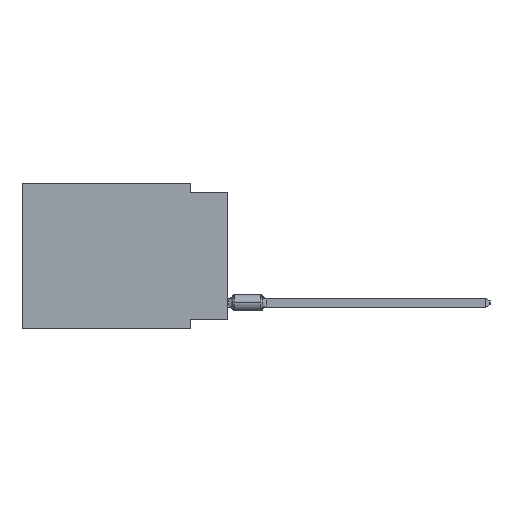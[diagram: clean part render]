
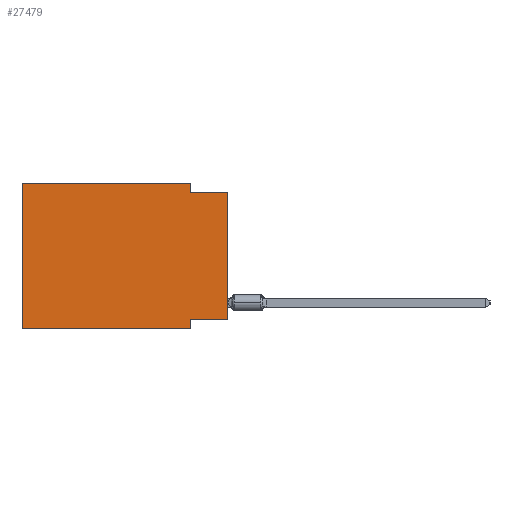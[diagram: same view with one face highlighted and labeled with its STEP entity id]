
A CAD part, left-side view. The second image highlights one B-rep face of the part: STEP entity #27479.
In plain terms, the highlighted planar face has unit normal (-1, 0, 0).
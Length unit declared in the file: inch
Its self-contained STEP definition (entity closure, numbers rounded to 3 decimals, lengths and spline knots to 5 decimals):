
#894 = VERTEX_POINT ( 'NONE', #2018 ) ;
#1038 = ORIENTED_EDGE ( 'NONE', *, *, #21300, .F. ) ;
#1044 = EDGE_CURVE ( 'NONE', #894, #15032, #33565, .T. ) ;
#1899 = DIRECTION ( 'NONE',  ( 0., -1., 0. ) ) ;
#1952 = LINE ( 'NONE', #21117, #22006 ) ;
#2018 = CARTESIAN_POINT ( 'NONE',  ( 0., 0.1, 0. ) ) ;
#2833 = EDGE_CURVE ( 'NONE', #34640, #15910, #15839, .T. ) ;
#4750 = VERTEX_POINT ( 'NONE', #22282 ) ;
#5182 = CARTESIAN_POINT ( 'NONE',  ( 0., 0.55, -0.39 ) ) ;
#5413 = DIRECTION ( 'NONE',  ( 0., 1., 0. ) ) ;
#6310 = VECTOR ( 'NONE', #17006, 39.37008 ) ;
#6360 = VECTOR ( 'NONE', #30102, 39.37008 ) ;
#6631 = CARTESIAN_POINT ( 'NONE',  ( 0., 0.55, 0. ) ) ;
#6799 = EDGE_CURVE ( 'NONE', #15032, #14918, #14564, .T. ) ;
#6900 = CARTESIAN_POINT ( 'NONE',  ( 0., 0.1, -0.39 ) ) ;
#7447 = VERTEX_POINT ( 'NONE', #28663 ) ;
#7668 = CARTESIAN_POINT ( 'NONE',  ( 0., 0.1, -0.365 ) ) ;
#8268 = ORIENTED_EDGE ( 'NONE', *, *, #36046, .F. ) ;
#8317 = LINE ( 'NONE', #19436, #23651 ) ;
#8436 = ORIENTED_EDGE ( 'NONE', *, *, #2833, .F. ) ;
#9381 = FACE_OUTER_BOUND ( 'NONE', #31543, .T. ) ;
#11258 = EDGE_CURVE ( 'NONE', #7447, #15910, #35103, .T. ) ;
#12214 = ORIENTED_EDGE ( 'NONE', *, *, #6799, .F. ) ;
#12831 = DIRECTION ( 'NONE',  ( 1., 0., 0. ) ) ;
#13081 = DIRECTION ( 'NONE',  ( 0., 0., 1. ) ) ;
#14133 = ORIENTED_EDGE ( 'NONE', *, *, #23412, .T. ) ;
#14235 = CARTESIAN_POINT ( 'NONE',  ( 0., 0.1, 0. ) ) ;
#14552 = VECTOR ( 'NONE', #5413, 39.37008 ) ;
#14564 = LINE ( 'NONE', #22567, #31024 ) ;
#14719 = CARTESIAN_POINT ( 'NONE',  ( 0., 0.55, 0. ) ) ;
#14918 = VERTEX_POINT ( 'NONE', #34698 ) ;
#15032 = VERTEX_POINT ( 'NONE', #18269 ) ;
#15839 = LINE ( 'NONE', #21483, #21558 ) ;
#15910 = VERTEX_POINT ( 'NONE', #6900 ) ;
#16382 = LINE ( 'NONE', #30757, #14552 ) ;
#17006 = DIRECTION ( 'NONE',  ( 0., -1., 0. ) ) ;
#18269 = CARTESIAN_POINT ( 'NONE',  ( 0., 0.1, -0.025 ) ) ;
#18277 = ORIENTED_EDGE ( 'NONE', *, *, #29697, .F. ) ;
#18295 = ORIENTED_EDGE ( 'NONE', *, *, #1044, .F. ) ;
#18969 = VECTOR ( 'NONE', #1899, 39.37008 ) ;
#19436 = CARTESIAN_POINT ( 'NONE',  ( 0., 0.55, 0. ) ) ;
#21117 = CARTESIAN_POINT ( 'NONE',  ( 0., 0., 0. ) ) ;
#21300 = EDGE_CURVE ( 'NONE', #7447, #21398, #8317, .T. ) ;
#21398 = VERTEX_POINT ( 'NONE', #14719 ) ;
#21483 = CARTESIAN_POINT ( 'NONE',  ( 0., 0.1, -0.39 ) ) ;
#21558 = VECTOR ( 'NONE', #23678, 39.37008 ) ;
#22006 = VECTOR ( 'NONE', #13081, 39.37008 ) ;
#22282 = CARTESIAN_POINT ( 'NONE',  ( 0., 0., -0.365 ) ) ;
#22567 = CARTESIAN_POINT ( 'NONE',  ( 0., 0., -0.025 ) ) ;
#23412 = EDGE_CURVE ( 'NONE', #4750, #14918, #1952, .T. ) ;
#23651 = VECTOR ( 'NONE', #30550, 39.37008 ) ;
#23678 = DIRECTION ( 'NONE',  ( 0., 0., -1. ) ) ;
#23954 = DIRECTION ( 'NONE',  ( 0., 0., -1. ) ) ;
#26150 = PLANE ( 'NONE',  #30141 ) ;
#27479 = ADVANCED_FACE ( 'NONE', ( #9381 ), #26150, .F. ) ;
#28299 = CARTESIAN_POINT ( 'NONE',  ( 0., 0.55, 0. ) ) ;
#28663 = CARTESIAN_POINT ( 'NONE',  ( 0., 0.55, -0.39 ) ) ;
#28825 = LINE ( 'NONE', #28299, #6310 ) ;
#29697 = EDGE_CURVE ( 'NONE', #4750, #34640, #16382, .T. ) ;
#30102 = DIRECTION ( 'NONE',  ( 0., 0., -1. ) ) ;
#30141 = AXIS2_PLACEMENT_3D ( 'NONE', #6631, #12831, #23954 ) ;
#30550 = DIRECTION ( 'NONE',  ( 0., 0., 1. ) ) ;
#30757 = CARTESIAN_POINT ( 'NONE',  ( 0., 0., -0.365 ) ) ;
#31024 = VECTOR ( 'NONE', #33697, 39.37008 ) ;
#31543 = EDGE_LOOP ( 'NONE', ( #14133, #12214, #18295, #8268, #1038, #34833, #8436, #18277 ) ) ;
#33565 = LINE ( 'NONE', #14235, #6360 ) ;
#33697 = DIRECTION ( 'NONE',  ( 0., -1., 0. ) ) ;
#34640 = VERTEX_POINT ( 'NONE', #7668 ) ;
#34698 = CARTESIAN_POINT ( 'NONE',  ( 0., 0., -0.025 ) ) ;
#34833 = ORIENTED_EDGE ( 'NONE', *, *, #11258, .T. ) ;
#35103 = LINE ( 'NONE', #5182, #18969 ) ;
#36046 = EDGE_CURVE ( 'NONE', #21398, #894, #28825, .T. ) ;
